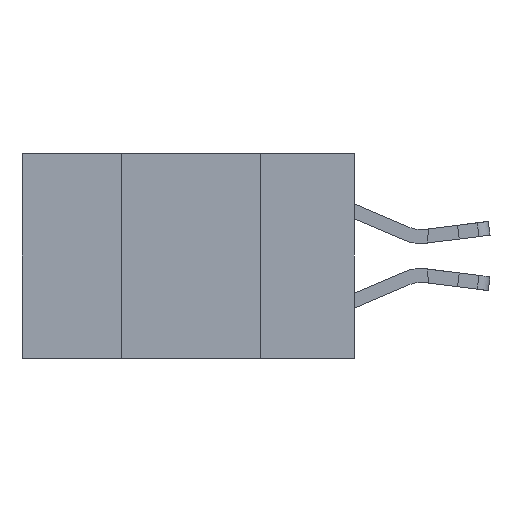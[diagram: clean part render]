
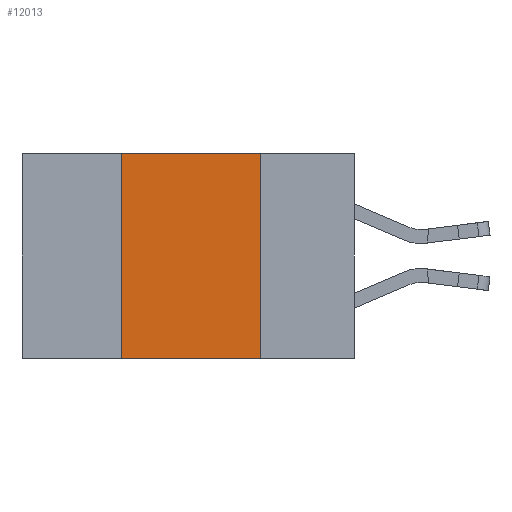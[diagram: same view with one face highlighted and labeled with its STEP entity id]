
A CAD part, left-side view. The second image highlights one B-rep face of the part: STEP entity #12013.
In plain terms, the highlighted planar face has unit normal (-1, 0, 0).
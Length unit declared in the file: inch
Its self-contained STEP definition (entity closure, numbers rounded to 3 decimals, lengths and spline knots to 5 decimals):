
#789 = ORIENTED_EDGE ( 'NONE', *, *, #12310, .F. ) ;
#827 = DIRECTION ( 'NONE',  ( 1., 0., 0. ) ) ;
#1573 = VECTOR ( 'NONE', #7436, 39.37008 ) ;
#1916 = CARTESIAN_POINT ( 'NONE',  ( 0., 0.42, 0. ) ) ;
#1943 = PLANE ( 'NONE',  #3139 ) ;
#2248 = VERTEX_POINT ( 'NONE', #1916 ) ;
#2310 = CARTESIAN_POINT ( 'NONE',  ( 0., 0.17, 0. ) ) ;
#2527 = EDGE_CURVE ( 'NONE', #4525, #9024, #3451, .T. ) ;
#3139 = AXIS2_PLACEMENT_3D ( 'NONE', #7289, #827, #8532 ) ;
#3451 = LINE ( 'NONE', #3512, #8390 ) ;
#3512 = CARTESIAN_POINT ( 'NONE',  ( 0., 0.6, -0.37 ) ) ;
#4208 = LINE ( 'NONE', #10678, #1573 ) ;
#4459 = EDGE_CURVE ( 'NONE', #11792, #9024, #12353, .T. ) ;
#4525 = VERTEX_POINT ( 'NONE', #6174 ) ;
#4701 = VECTOR ( 'NONE', #9236, 39.37008 ) ;
#4890 = CARTESIAN_POINT ( 'NONE',  ( 0., 0.42, -0.37 ) ) ;
#5296 = ORIENTED_EDGE ( 'NONE', *, *, #4459, .F. ) ;
#6174 = CARTESIAN_POINT ( 'NONE',  ( 0., 0.42, -0.37 ) ) ;
#7289 = CARTESIAN_POINT ( 'NONE',  ( 0., 0.6, 0. ) ) ;
#7436 = DIRECTION ( 'NONE',  ( 0., -1., 0. ) ) ;
#7791 = DIRECTION ( 'NONE',  ( 0., -1., 0. ) ) ;
#7957 = CARTESIAN_POINT ( 'NONE',  ( 0., 0.17, -0.37 ) ) ;
#8390 = VECTOR ( 'NONE', #7791, 39.37008 ) ;
#8532 = DIRECTION ( 'NONE',  ( 0., 0., -1. ) ) ;
#8938 = DIRECTION ( 'NONE',  ( 0., 0., 1. ) ) ;
#8989 = ORIENTED_EDGE ( 'NONE', *, *, #2527, .T. ) ;
#9024 = VERTEX_POINT ( 'NONE', #7957 ) ;
#9165 = CARTESIAN_POINT ( 'NONE',  ( 0., 0.17, -0.37 ) ) ;
#9236 = DIRECTION ( 'NONE',  ( 0., 0., -1. ) ) ;
#9513 = EDGE_LOOP ( 'NONE', ( #5296, #10081, #789, #8989 ) ) ;
#10081 = ORIENTED_EDGE ( 'NONE', *, *, #11603, .F. ) ;
#10678 = CARTESIAN_POINT ( 'NONE',  ( 0., 0.6, 0. ) ) ;
#11587 = VECTOR ( 'NONE', #8938, 39.37008 ) ;
#11603 = EDGE_CURVE ( 'NONE', #2248, #11792, #4208, .T. ) ;
#11792 = VERTEX_POINT ( 'NONE', #2310 ) ;
#12013 = ADVANCED_FACE ( 'NONE', ( #12761 ), #1943, .F. ) ;
#12263 = LINE ( 'NONE', #4890, #11587 ) ;
#12310 = EDGE_CURVE ( 'NONE', #4525, #2248, #12263, .T. ) ;
#12353 = LINE ( 'NONE', #9165, #4701 ) ;
#12761 = FACE_OUTER_BOUND ( 'NONE', #9513, .T. ) ;
